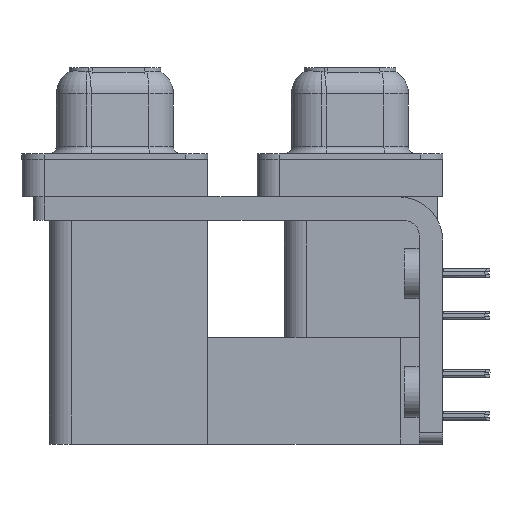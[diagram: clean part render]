
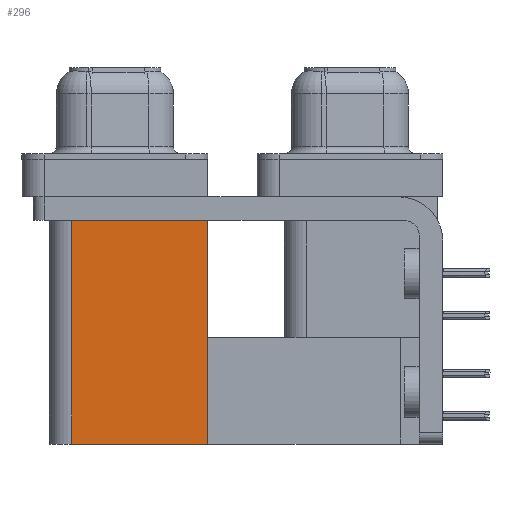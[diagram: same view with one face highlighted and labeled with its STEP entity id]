
A CAD part, left-side view. The second image highlights one B-rep face of the part: STEP entity #296.
In plain terms, the highlighted planar face has unit normal (-1, 0, 0).
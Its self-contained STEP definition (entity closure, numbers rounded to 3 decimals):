
#296 = ADVANCED_FACE ( 'NONE', ( #15952 ), #5060, .F. ) ;
#1001 = VERTEX_POINT ( 'NONE', #25482 ) ;
#3121 = AXIS2_PLACEMENT_3D ( 'NONE', #11992, #30997, #16430 ) ;
#5060 = PLANE ( 'NONE',  #3121 ) ;
#5177 = DIRECTION ( 'NONE',  ( 0., 0., 1. ) ) ;
#5355 = ORIENTED_EDGE ( 'NONE', *, *, #34940, .T. ) ;
#10888 = VERTEX_POINT ( 'NONE', #13909 ) ;
#11277 = DIRECTION ( 'NONE',  ( 0., 0., 1. ) ) ;
#11992 = CARTESIAN_POINT ( 'NONE',  ( 3.765, 9.6, -19.2 ) ) ;
#12717 = CARTESIAN_POINT ( 'NONE',  ( 3.765, 9.6, -19.2 ) ) ;
#13227 = EDGE_CURVE ( 'NONE', #1001, #10888, #27052, .T. ) ;
#13345 = CARTESIAN_POINT ( 'NONE',  ( 3.765, 18.8, -19.2 ) ) ;
#13754 = VECTOR ( 'NONE', #15682, 1000. ) ;
#13909 = CARTESIAN_POINT ( 'NONE',  ( 3.765, 18.8, -19.2 ) ) ;
#14965 = CARTESIAN_POINT ( 'NONE',  ( 3.765, 9.6, -2.5 ) ) ;
#15682 = DIRECTION ( 'NONE',  ( 0., 1., 0. ) ) ;
#15952 = FACE_OUTER_BOUND ( 'NONE', #30464, .T. ) ;
#16430 = DIRECTION ( 'NONE',  ( 0., 0., -1. ) ) ;
#18923 = ORIENTED_EDGE ( 'NONE', *, *, #21481, .T. ) ;
#19630 = CARTESIAN_POINT ( 'NONE',  ( 3.765, 18.8, -2.5 ) ) ;
#20308 = ORIENTED_EDGE ( 'NONE', *, *, #13227, .F. ) ;
#21481 = EDGE_CURVE ( 'NONE', #27899, #33507, #23095, .T. ) ;
#23095 = LINE ( 'NONE', #14965, #13754 ) ;
#25482 = CARTESIAN_POINT ( 'NONE',  ( 3.765, 9.6, -19.2 ) ) ;
#27052 = LINE ( 'NONE', #12717, #37498 ) ;
#27899 = VERTEX_POINT ( 'NONE', #47077 ) ;
#30464 = EDGE_LOOP ( 'NONE', ( #18923, #46235, #20308, #5355 ) ) ;
#30997 = DIRECTION ( 'NONE',  ( 1., 0., 0. ) ) ;
#33507 = VERTEX_POINT ( 'NONE', #19630 ) ;
#34940 = EDGE_CURVE ( 'NONE', #1001, #27899, #48816, .T. ) ;
#35494 = EDGE_CURVE ( 'NONE', #10888, #33507, #43458, .T. ) ;
#37498 = VECTOR ( 'NONE', #41606, 1000. ) ;
#38022 = VECTOR ( 'NONE', #11277, 1000. ) ;
#41606 = DIRECTION ( 'NONE',  ( 0., 1., 0. ) ) ;
#43458 = LINE ( 'NONE', #13345, #45962 ) ;
#45120 = CARTESIAN_POINT ( 'NONE',  ( 3.765, 9.6, -19.2 ) ) ;
#45962 = VECTOR ( 'NONE', #5177, 1000. ) ;
#46235 = ORIENTED_EDGE ( 'NONE', *, *, #35494, .F. ) ;
#47077 = CARTESIAN_POINT ( 'NONE',  ( 3.765, 9.6, -2.5 ) ) ;
#48816 = LINE ( 'NONE', #45120, #38022 ) ;
